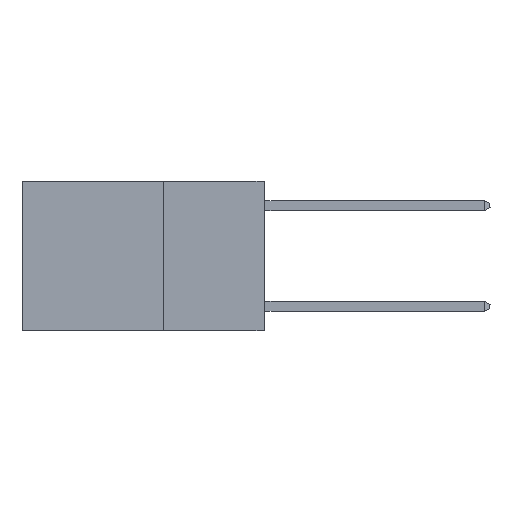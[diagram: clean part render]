
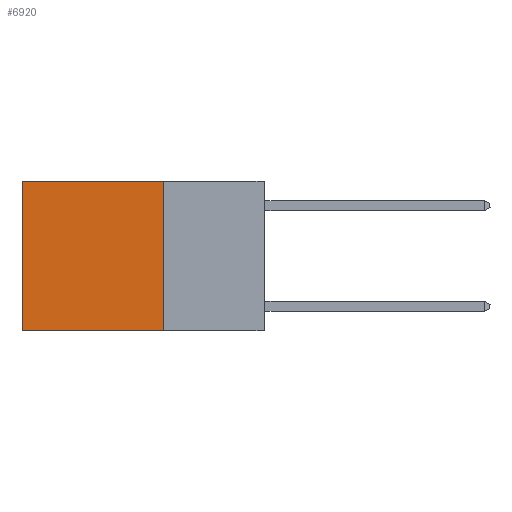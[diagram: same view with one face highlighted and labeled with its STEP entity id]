
A CAD part, left-side view. The second image highlights one B-rep face of the part: STEP entity #6920.
In plain terms, the highlighted planar face has unit normal (-1, 0, 0).
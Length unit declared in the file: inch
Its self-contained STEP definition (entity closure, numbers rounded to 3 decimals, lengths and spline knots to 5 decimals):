
#1029 = VERTEX_POINT ( 'NONE', #26209 ) ;
#1151 = CARTESIAN_POINT ( 'NONE',  ( 0.2625, 0.6, 0. ) ) ;
#1676 = ORIENTED_EDGE ( 'NONE', *, *, #3201, .T. ) ;
#3201 = EDGE_CURVE ( 'NONE', #4152, #25944, #18676, .T. ) ;
#3261 = CARTESIAN_POINT ( 'NONE',  ( 0.2625, 0.25, 0. ) ) ;
#4113 = EDGE_LOOP ( 'NONE', ( #1676, #23608, #4150, #8998 ) ) ;
#4150 = ORIENTED_EDGE ( 'NONE', *, *, #13489, .F. ) ;
#4152 = VERTEX_POINT ( 'NONE', #25260 ) ;
#4433 = EDGE_CURVE ( 'NONE', #1029, #4152, #18129, .T. ) ;
#4554 = VERTEX_POINT ( 'NONE', #13542 ) ;
#5584 = VECTOR ( 'NONE', #10223, 39.37008 ) ;
#6920 = ADVANCED_FACE ( 'NONE', ( #21929 ), #7172, .F. ) ;
#7172 = PLANE ( 'NONE',  #24937 ) ;
#7309 = DIRECTION ( 'NONE',  ( 0., 0., -1. ) ) ;
#8998 = ORIENTED_EDGE ( 'NONE', *, *, #4433, .T. ) ;
#9943 = CARTESIAN_POINT ( 'NONE',  ( 0.2625, 0.25, 0. ) ) ;
#10223 = DIRECTION ( 'NONE',  ( 0., 0., -1. ) ) ;
#10400 = EDGE_CURVE ( 'NONE', #4554, #25944, #12276, .T. ) ;
#10465 = VECTOR ( 'NONE', #11464, 39.37008 ) ;
#11464 = DIRECTION ( 'NONE',  ( 0., 1., 0. ) ) ;
#12276 = LINE ( 'NONE', #18255, #20620 ) ;
#13441 = CARTESIAN_POINT ( 'NONE',  ( 0.2625, 0.25, 0. ) ) ;
#13489 = EDGE_CURVE ( 'NONE', #1029, #4554, #25104, .T. ) ;
#13542 = CARTESIAN_POINT ( 'NONE',  ( 0.2625, 0.25, -0.37 ) ) ;
#15664 = DIRECTION ( 'NONE',  ( 1., 0., 0. ) ) ;
#15810 = VECTOR ( 'NONE', #22702, 39.37008 ) ;
#18129 = LINE ( 'NONE', #3261, #10465 ) ;
#18255 = CARTESIAN_POINT ( 'NONE',  ( 0.2625, 0.25, -0.37 ) ) ;
#18676 = LINE ( 'NONE', #1151, #15810 ) ;
#20620 = VECTOR ( 'NONE', #26751, 39.37008 ) ;
#20646 = CARTESIAN_POINT ( 'NONE',  ( 0.2625, 0.6, -0.37 ) ) ;
#21929 = FACE_OUTER_BOUND ( 'NONE', #4113, .T. ) ;
#22702 = DIRECTION ( 'NONE',  ( 0., 0., -1. ) ) ;
#23608 = ORIENTED_EDGE ( 'NONE', *, *, #10400, .F. ) ;
#24937 = AXIS2_PLACEMENT_3D ( 'NONE', #13441, #15664, #7309 ) ;
#25104 = LINE ( 'NONE', #9943, #5584 ) ;
#25260 = CARTESIAN_POINT ( 'NONE',  ( 0.2625, 0.6, 0. ) ) ;
#25944 = VERTEX_POINT ( 'NONE', #20646 ) ;
#26209 = CARTESIAN_POINT ( 'NONE',  ( 0.2625, 0.25, 0. ) ) ;
#26751 = DIRECTION ( 'NONE',  ( 0., 1., 0. ) ) ;
